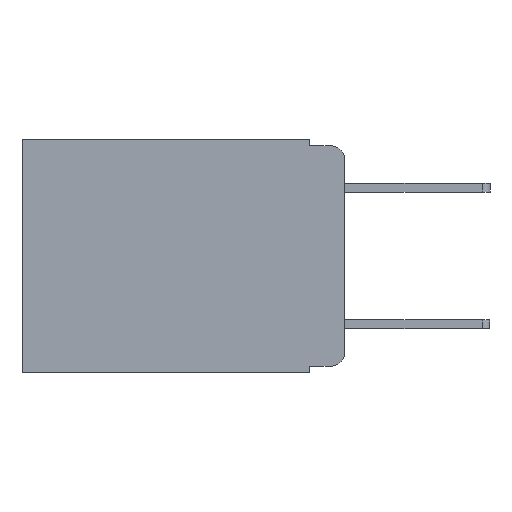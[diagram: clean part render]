
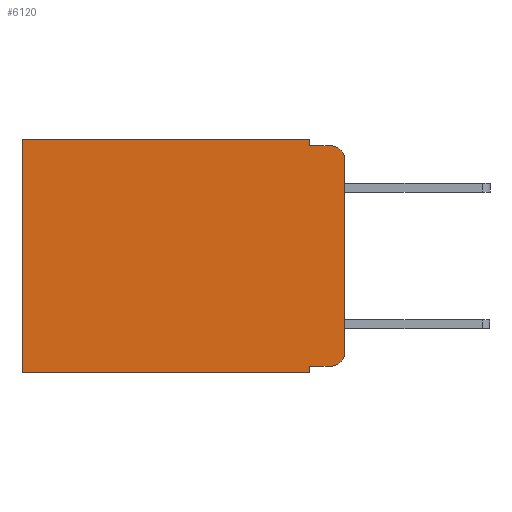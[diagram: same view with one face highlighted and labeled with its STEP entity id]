
A CAD part, left-side view. The second image highlights one B-rep face of the part: STEP entity #6120.
In plain terms, the highlighted planar face has unit normal (-1, 0, 0).
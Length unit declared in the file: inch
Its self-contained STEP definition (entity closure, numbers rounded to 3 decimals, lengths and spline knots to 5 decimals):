
#325 = ORIENTED_EDGE ( 'NONE', *, *, #1196, .T. ) ;
#449 = VERTEX_POINT ( 'NONE', #10152 ) ;
#525 = EDGE_CURVE ( 'NONE', #8410, #4564, #706, .T. ) ;
#706 = CIRCLE ( 'NONE', #2196, 0.02 ) ;
#906 = AXIS2_PLACEMENT_3D ( 'NONE', #9078, #6836, #1816 ) ;
#1099 = DIRECTION ( 'NONE',  ( 0., 1., 0. ) ) ;
#1178 = DIRECTION ( 'NONE',  ( 0., -1., 0. ) ) ;
#1196 = EDGE_CURVE ( 'NONE', #5408, #8410, #9913, .T. ) ;
#1327 = VERTEX_POINT ( 'NONE', #1706 ) ;
#1466 = CARTESIAN_POINT ( 'NONE',  ( 0.298, 0.02, -0.03 ) ) ;
#1494 = CARTESIAN_POINT ( 'NONE',  ( 0.298, 0.051, -0.01 ) ) ;
#1501 = CARTESIAN_POINT ( 'NONE',  ( 0.298, 0.051, -0.333 ) ) ;
#1660 = EDGE_LOOP ( 'NONE', ( #1854, #8703, #7256, #2915, #6531, #5912, #2429, #6314, #325, #7478 ) ) ;
#1706 = CARTESIAN_POINT ( 'NONE',  ( 0.298, 0., -0.03 ) ) ;
#1734 = CARTESIAN_POINT ( 'NONE',  ( 0.298, 0.473, -0.343 ) ) ;
#1816 = DIRECTION ( 'NONE',  ( 0., 0., -1. ) ) ;
#1817 = EDGE_CURVE ( 'NONE', #5408, #7630, #6741, .T. ) ;
#1854 = ORIENTED_EDGE ( 'NONE', *, *, #8784, .F. ) ;
#2167 = DIRECTION ( 'NONE',  ( 0., 0., -1. ) ) ;
#2196 = AXIS2_PLACEMENT_3D ( 'NONE', #9186, #5665, #9656 ) ;
#2267 = CARTESIAN_POINT ( 'NONE',  ( 0.298, 0.051, 0. ) ) ;
#2389 = DIRECTION ( 'NONE',  ( 0., 0., -1. ) ) ;
#2398 = DIRECTION ( 'NONE',  ( 0., 0., -1. ) ) ;
#2429 = ORIENTED_EDGE ( 'NONE', *, *, #4452, .F. ) ;
#2548 = DIRECTION ( 'NONE',  ( 0., 0., -1. ) ) ;
#2679 = VECTOR ( 'NONE', #1178, 39.37008 ) ;
#2705 = CARTESIAN_POINT ( 'NONE',  ( 0.298, 0.473, 0. ) ) ;
#2751 = DIRECTION ( 'NONE',  ( 0., 1., 0. ) ) ;
#2915 = ORIENTED_EDGE ( 'NONE', *, *, #4226, .F. ) ;
#3048 = EDGE_CURVE ( 'NONE', #4292, #7738, #10583, .T. ) ;
#3230 = CARTESIAN_POINT ( 'NONE',  ( 0.298, 0., -0.343 ) ) ;
#3603 = CARTESIAN_POINT ( 'NONE',  ( 0.298, 0., 0. ) ) ;
#3667 = EDGE_CURVE ( 'NONE', #6854, #4292, #5321, .T. ) ;
#3957 = LINE ( 'NONE', #3230, #5811 ) ;
#3989 = DIRECTION ( 'NONE',  ( 0., 0., -1. ) ) ;
#4090 = CARTESIAN_POINT ( 'NONE',  ( 0.298, 0.051, 0. ) ) ;
#4226 = EDGE_CURVE ( 'NONE', #6854, #449, #9977, .T. ) ;
#4292 = VERTEX_POINT ( 'NONE', #2705 ) ;
#4452 = EDGE_CURVE ( 'NONE', #7630, #7738, #3957, .T. ) ;
#4502 = VECTOR ( 'NONE', #2167, 39.37008 ) ;
#4564 = VERTEX_POINT ( 'NONE', #9680 ) ;
#4628 = CARTESIAN_POINT ( 'NONE',  ( 0.298, 0.02, -0.333 ) ) ;
#4761 = EDGE_CURVE ( 'NONE', #449, #8127, #9045, .T. ) ;
#5321 = LINE ( 'NONE', #3603, #7181 ) ;
#5408 = VERTEX_POINT ( 'NONE', #1501 ) ;
#5486 = CARTESIAN_POINT ( 'NONE',  ( 0.298, 0.051, 0. ) ) ;
#5665 = DIRECTION ( 'NONE',  ( -1., 0., 0. ) ) ;
#5811 = VECTOR ( 'NONE', #1099, 39.37008 ) ;
#5871 = CARTESIAN_POINT ( 'NONE',  ( 0.298, 0., 0. ) ) ;
#5912 = ORIENTED_EDGE ( 'NONE', *, *, #3048, .T. ) ;
#5946 = VECTOR ( 'NONE', #2389, 39.37008 ) ;
#6012 = PLANE ( 'NONE',  #906 ) ;
#6120 = ADVANCED_FACE ( 'NONE', ( #6597 ), #6012, .F. ) ;
#6238 = CARTESIAN_POINT ( 'NONE',  ( 0.298, 0.051, -0.333 ) ) ;
#6314 = ORIENTED_EDGE ( 'NONE', *, *, #1817, .F. ) ;
#6321 = LINE ( 'NONE', #5871, #8115 ) ;
#6531 = ORIENTED_EDGE ( 'NONE', *, *, #3667, .T. ) ;
#6570 = CARTESIAN_POINT ( 'NONE',  ( 0.298, 0.051, -0.343 ) ) ;
#6593 = AXIS2_PLACEMENT_3D ( 'NONE', #1466, #7313, #2398 ) ;
#6597 = FACE_OUTER_BOUND ( 'NONE', #1660, .T. ) ;
#6741 = LINE ( 'NONE', #4090, #10475 ) ;
#6836 = DIRECTION ( 'NONE',  ( 1., 0., 0. ) ) ;
#6854 = VERTEX_POINT ( 'NONE', #5486 ) ;
#7181 = VECTOR ( 'NONE', #2751, 39.37008 ) ;
#7256 = ORIENTED_EDGE ( 'NONE', *, *, #4761, .F. ) ;
#7266 = CIRCLE ( 'NONE', #6593, 0.02 ) ;
#7313 = DIRECTION ( 'NONE',  ( -1., 0., 0. ) ) ;
#7478 = ORIENTED_EDGE ( 'NONE', *, *, #525, .T. ) ;
#7630 = VERTEX_POINT ( 'NONE', #6570 ) ;
#7738 = VERTEX_POINT ( 'NONE', #1734 ) ;
#7961 = VECTOR ( 'NONE', #9761, 39.37008 ) ;
#8115 = VECTOR ( 'NONE', #2548, 39.37008 ) ;
#8127 = VERTEX_POINT ( 'NONE', #8846 ) ;
#8410 = VERTEX_POINT ( 'NONE', #4628 ) ;
#8666 = EDGE_CURVE ( 'NONE', #1327, #8127, #7266, .T. ) ;
#8703 = ORIENTED_EDGE ( 'NONE', *, *, #8666, .T. ) ;
#8784 = EDGE_CURVE ( 'NONE', #1327, #4564, #6321, .T. ) ;
#8846 = CARTESIAN_POINT ( 'NONE',  ( 0.298, 0.02, -0.01 ) ) ;
#9045 = LINE ( 'NONE', #1494, #2679 ) ;
#9078 = CARTESIAN_POINT ( 'NONE',  ( 0.298, 0., 0. ) ) ;
#9186 = CARTESIAN_POINT ( 'NONE',  ( 0.298, 0.02, -0.313 ) ) ;
#9641 = CARTESIAN_POINT ( 'NONE',  ( 0.298, 0.473, 0. ) ) ;
#9656 = DIRECTION ( 'NONE',  ( 0., 0., -1. ) ) ;
#9680 = CARTESIAN_POINT ( 'NONE',  ( 0.298, 0., -0.313 ) ) ;
#9761 = DIRECTION ( 'NONE',  ( 0., -1., 0. ) ) ;
#9913 = LINE ( 'NONE', #6238, #7961 ) ;
#9977 = LINE ( 'NONE', #2267, #5946 ) ;
#10152 = CARTESIAN_POINT ( 'NONE',  ( 0.298, 0.051, -0.01 ) ) ;
#10475 = VECTOR ( 'NONE', #3989, 39.37008 ) ;
#10583 = LINE ( 'NONE', #9641, #4502 ) ;
